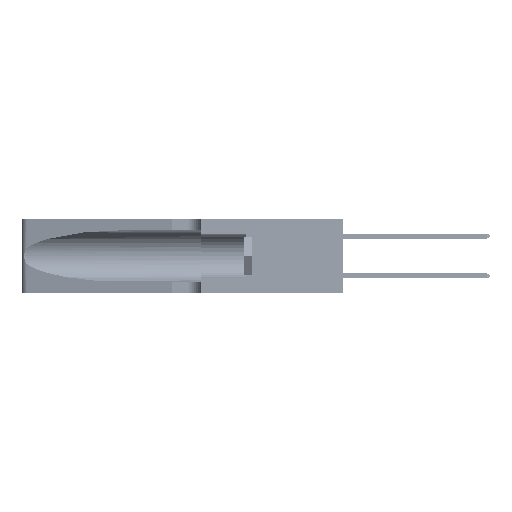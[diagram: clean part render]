
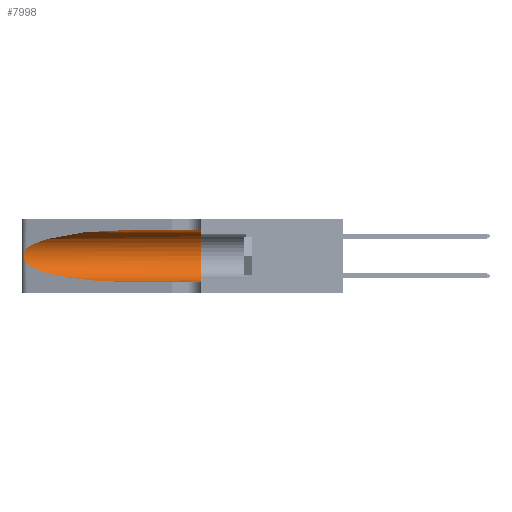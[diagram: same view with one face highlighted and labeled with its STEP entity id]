
A CAD part, left-side view. The second image highlights one B-rep face of the part: STEP entity #7998.
In plain terms, the highlighted cylindrical face has radius 3.308 mm (diameter 6.617 mm), a partial arc.
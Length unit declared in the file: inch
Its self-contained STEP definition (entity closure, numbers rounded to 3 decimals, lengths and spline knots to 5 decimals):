
#613 = EDGE_CURVE ( 'NONE', #2941, #29343, #12651, .T. ) ;
#1159 = ORIENTED_EDGE ( 'NONE', *, *, #41061, .T. ) ;
#2861 = CARTESIAN_POINT ( 'NONE',  ( 0.25555, 1.22994, 0.2215 ) ) ;
#2941 = VERTEX_POINT ( 'NONE', #28161 ) ;
#3077 = EDGE_CURVE ( 'NONE', #33556, #34856, #45130, .T. ) ;
#4399 = CARTESIAN_POINT ( 'NONE',  ( 0.1305, 1.61858, 0.05475 ) ) ;
#5222 = CARTESIAN_POINT ( 'NONE',  ( 0.1305, 0.35, 0.05475 ) ) ;
#5941 = CARTESIAN_POINT ( 'NONE',  ( 0.1305, 0.72297, 0.05475 ) ) ;
#7998 = ADVANCED_FACE ( 'NONE', ( #46620 ), #20902, .F. ) ;
#9687 = EDGE_CURVE ( 'NONE', #29343, #33556, #31632, .T. ) ;
#10116 = DIRECTION ( 'NONE',  ( 0., 0., -1. ) ) ;
#10401 = CARTESIAN_POINT ( 'NONE',  ( 0.25487, 1.22718, 0.22369 ) ) ;
#11176 = CARTESIAN_POINT ( 'NONE',  ( 0.1305, 0.72297, 0.31525 ) ) ;
#12639 = VERTEX_POINT ( 'NONE', #44677 ) ;
#12651 =( BOUNDED_CURVE ( )  B_SPLINE_CURVE ( 3, ( #11176, #18535, #38424, #14878 ),
 .UNSPECIFIED., .F., .F. ) 
 B_SPLINE_CURVE_WITH_KNOTS ( ( 4, 4 ),
 ( 1.5708, 2.84003 ),
 .UNSPECIFIED. ) 
 CURVE ( )  GEOMETRIC_REPRESENTATION_ITEM ( )  RATIONAL_B_SPLINE_CURVE ( ( 1., 0.87, 0.87, 1. ) ) 
 REPRESENTATION_ITEM ( '' )  );
#14018 = ORIENTED_EDGE ( 'NONE', *, *, #9687, .T. ) ;
#14762 = CARTESIAN_POINT ( 'NONE',  ( 0.25487, 1.22718, 0.14631 ) ) ;
#14878 = CARTESIAN_POINT ( 'NONE',  ( 0.25487, 1.22718, 0.22369 ) ) ;
#15023 = VECTOR ( 'NONE', #34451, 39.37008 ) ;
#15687 = ORIENTED_EDGE ( 'NONE', *, *, #33722, .F. ) ;
#16193 = CARTESIAN_POINT ( 'NONE',  ( 0.25487, 1.22718, 0.22369 ) ) ;
#17099 = AXIS2_PLACEMENT_3D ( 'NONE', #21319, #40670, #10116 ) ;
#17574 = CARTESIAN_POINT ( 'NONE',  ( 0.1305, 0.72297, 0.05475 ) ) ;
#18535 = CARTESIAN_POINT ( 'NONE',  ( 0.18966, 0.96281, 0.31525 ) ) ;
#19994 = VECTOR ( 'NONE', #20306, 39.37008 ) ;
#20296 = DIRECTION ( 'NONE',  ( 0., 1., 0. ) ) ;
#20306 = DIRECTION ( 'NONE',  ( 0., -1., 0. ) ) ;
#20755 = CARTESIAN_POINT ( 'NONE',  ( 0.1305, 0.35, 0.185 ) ) ;
#20902 = CYLINDRICAL_SURFACE ( 'NONE', #17099, 0.13025 ) ;
#21319 = CARTESIAN_POINT ( 'NONE',  ( 0.1305, 1.61858, 0.185 ) ) ;
#21352 = CARTESIAN_POINT ( 'NONE',  ( 0.18966, 0.96281, 0.05475 ) ) ;
#24826 = CARTESIAN_POINT ( 'NONE',  ( 0.2373, 1.15595, 0.08982 ) ) ;
#24920 = EDGE_LOOP ( 'NONE', ( #29334, #14018, #31514, #1159, #15687, #35566 ) ) ;
#25152 = LINE ( 'NONE', #26601, #15023 ) ;
#25772 = CARTESIAN_POINT ( 'NONE',  ( 0.26075, 1.23896, 0.178 ) ) ;
#26088 = CARTESIAN_POINT ( 'NONE',  ( 0.26017, 1.23833, 0.17102 ) ) ;
#26601 = CARTESIAN_POINT ( 'NONE',  ( 0.1305, 1.61858, 0.31525 ) ) ;
#28161 = CARTESIAN_POINT ( 'NONE',  ( 0.1305, 0.72297, 0.31525 ) ) ;
#28243 = AXIS2_PLACEMENT_3D ( 'NONE', #20755, #20296, #31934 ) ;
#29334 = ORIENTED_EDGE ( 'NONE', *, *, #613, .T. ) ;
#29343 = VERTEX_POINT ( 'NONE', #16193 ) ;
#29450 = CARTESIAN_POINT ( 'NONE',  ( 0.25789, 1.23486, 0.15765 ) ) ;
#29608 = CARTESIAN_POINT ( 'NONE',  ( 0.25555, 1.22993, 0.14849 ) ) ;
#29936 = CARTESIAN_POINT ( 'NONE',  ( 0.25854, 1.2359, 0.20912 ) ) ;
#31514 = ORIENTED_EDGE ( 'NONE', *, *, #3077, .T. ) ;
#31632 = B_SPLINE_CURVE_WITH_KNOTS ( 'NONE', 3,
 ( #10401, #2861, #48704, #37651, #29936, #44847, #37822, #25772, #26088, #37320, #29450, #41146, #29608, #14762 ),
 .UNSPECIFIED., .F., .F.,
 ( 4, 2, 2, 2, 2, 2, 4 ),
 ( 0., 0.00027, 0.00053, 0.00107, 0.0016, 0.00187, 0.00214 ),
 .UNSPECIFIED. ) ;
#31934 = DIRECTION ( 'NONE',  ( 0., 0., 1. ) ) ;
#32838 = CARTESIAN_POINT ( 'NONE',  ( 0.25487, 1.22718, 0.14631 ) ) ;
#33556 = VERTEX_POINT ( 'NONE', #42326 ) ;
#33722 = EDGE_CURVE ( 'NONE', #12639, #34110, #45800, .T. ) ;
#34110 = VERTEX_POINT ( 'NONE', #5222 ) ;
#34451 = DIRECTION ( 'NONE',  ( 0., -1., 0. ) ) ;
#34856 = VERTEX_POINT ( 'NONE', #17574 ) ;
#35566 = ORIENTED_EDGE ( 'NONE', *, *, #36509, .F. ) ;
#36509 = EDGE_CURVE ( 'NONE', #2941, #12639, #25152, .T. ) ;
#37320 = CARTESIAN_POINT ( 'NONE',  ( 0.25856, 1.23593, 0.16098 ) ) ;
#37651 = CARTESIAN_POINT ( 'NONE',  ( 0.25787, 1.23484, 0.2124 ) ) ;
#37822 = CARTESIAN_POINT ( 'NONE',  ( 0.26075, 1.23896, 0.19203 ) ) ;
#38424 = CARTESIAN_POINT ( 'NONE',  ( 0.2373, 1.15595, 0.28018 ) ) ;
#40670 = DIRECTION ( 'NONE',  ( 0., -1., 0. ) ) ;
#41061 = EDGE_CURVE ( 'NONE', #34856, #34110, #43901, .T. ) ;
#41146 = CARTESIAN_POINT ( 'NONE',  ( 0.25639, 1.23186, 0.15144 ) ) ;
#42326 = CARTESIAN_POINT ( 'NONE',  ( 0.25487, 1.22718, 0.14631 ) ) ;
#43901 = LINE ( 'NONE', #4399, #19994 ) ;
#44677 = CARTESIAN_POINT ( 'NONE',  ( 0.1305, 0.35, 0.31525 ) ) ;
#44847 = CARTESIAN_POINT ( 'NONE',  ( 0.26018, 1.23835, 0.19895 ) ) ;
#45130 =( BOUNDED_CURVE ( )  B_SPLINE_CURVE ( 3, ( #32838, #24826, #21352, #5941 ),
 .UNSPECIFIED., .F., .F. ) 
 B_SPLINE_CURVE_WITH_KNOTS ( ( 4, 4 ),
 ( 3.44316, 4.71239 ),
 .UNSPECIFIED. ) 
 CURVE ( )  GEOMETRIC_REPRESENTATION_ITEM ( )  RATIONAL_B_SPLINE_CURVE ( ( 1., 0.87, 0.87, 1. ) ) 
 REPRESENTATION_ITEM ( '' )  );
#45800 = CIRCLE ( 'NONE', #28243, 0.13025 ) ;
#46620 = FACE_OUTER_BOUND ( 'NONE', #24920, .T. ) ;
#48704 = CARTESIAN_POINT ( 'NONE',  ( 0.25639, 1.23184, 0.21858 ) ) ;
